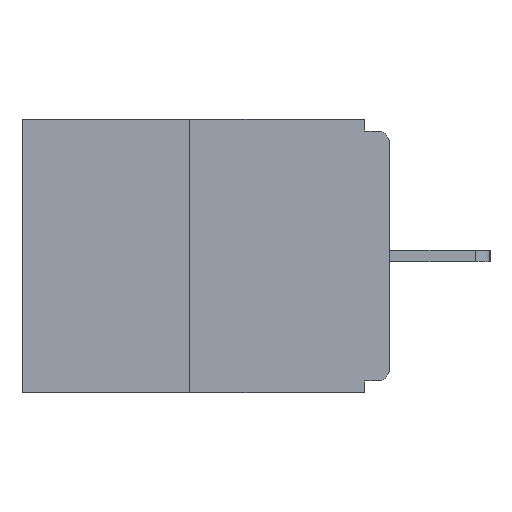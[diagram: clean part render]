
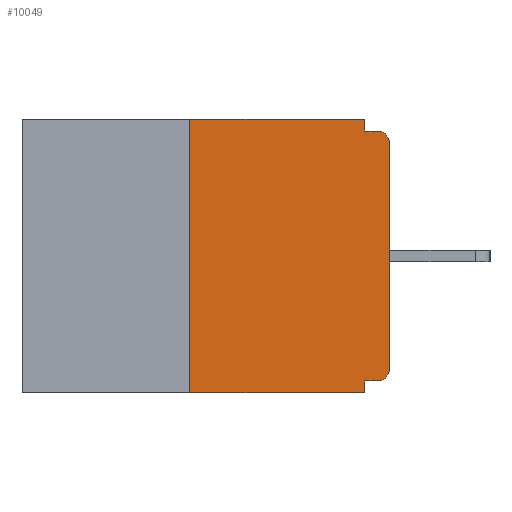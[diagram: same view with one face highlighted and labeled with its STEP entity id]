
A CAD part, left-side view. The second image highlights one B-rep face of the part: STEP entity #10049.
In plain terms, the highlighted planar face has unit normal (-1, 0, 0).
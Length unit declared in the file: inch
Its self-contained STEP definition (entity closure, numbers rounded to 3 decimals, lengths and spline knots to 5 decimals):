
#262 = LINE ( 'NONE', #20866, #19923 ) ;
#409 = EDGE_CURVE ( 'NONE', #17073, #11513, #262, .T. ) ;
#570 = CARTESIAN_POINT ( 'NONE',  ( 0., 0.015, -0.015 ) ) ;
#1238 = CARTESIAN_POINT ( 'NONE',  ( 0., 0.25, 0. ) ) ;
#2079 = LINE ( 'NONE', #9654, #21127 ) ;
#2628 = ORIENTED_EDGE ( 'NONE', *, *, #21669, .F. ) ;
#2881 = CARTESIAN_POINT ( 'NONE',  ( 0., 0.031, -0.343 ) ) ;
#2946 = AXIS2_PLACEMENT_3D ( 'NONE', #9299, #22091, #11186 ) ;
#3404 = DIRECTION ( 'NONE',  ( 0., 0., -1. ) ) ;
#3660 = LINE ( 'NONE', #16465, #13060 ) ;
#4600 = DIRECTION ( 'NONE',  ( 0., -1., 0. ) ) ;
#4614 = EDGE_CURVE ( 'NONE', #7440, #17073, #14393, .T. ) ;
#5332 = DIRECTION ( 'NONE',  ( 0., -1., 0. ) ) ;
#5369 = DIRECTION ( 'NONE',  ( 0., -1., 0. ) ) ;
#6088 = CARTESIAN_POINT ( 'NONE',  ( 0., 0., -0.313 ) ) ;
#6449 = CARTESIAN_POINT ( 'NONE',  ( 0., 0.031, -0.015 ) ) ;
#6926 = CARTESIAN_POINT ( 'NONE',  ( 0., 0.031, 0. ) ) ;
#7405 = EDGE_CURVE ( 'NONE', #10400, #9303, #20586, .T. ) ;
#7440 = VERTEX_POINT ( 'NONE', #12117 ) ;
#7557 = VERTEX_POINT ( 'NONE', #8673 ) ;
#7775 = LINE ( 'NONE', #13926, #21281 ) ;
#7869 = ORIENTED_EDGE ( 'NONE', *, *, #21294, .T. ) ;
#8654 = CARTESIAN_POINT ( 'NONE',  ( 0., 0.031, -0.328 ) ) ;
#8673 = CARTESIAN_POINT ( 'NONE',  ( 0., 0., -0.03 ) ) ;
#8986 = EDGE_CURVE ( 'NONE', #15023, #16984, #2079, .T. ) ;
#9113 = CARTESIAN_POINT ( 'NONE',  ( 0., 0.46, 0. ) ) ;
#9299 = CARTESIAN_POINT ( 'NONE',  ( 0., 0.015, -0.313 ) ) ;
#9303 = VERTEX_POINT ( 'NONE', #1238 ) ;
#9559 = DIRECTION ( 'NONE',  ( -1., 0., 0. ) ) ;
#9654 = CARTESIAN_POINT ( 'NONE',  ( 0., 0.031, 0. ) ) ;
#10049 = ADVANCED_FACE ( 'NONE', ( #13450 ), #19945, .F. ) ;
#10400 = VERTEX_POINT ( 'NONE', #11899 ) ;
#10853 = ORIENTED_EDGE ( 'NONE', *, *, #8986, .F. ) ;
#10904 = VECTOR ( 'NONE', #13775, 39.37008 ) ;
#11186 = DIRECTION ( 'NONE',  ( 0., 0., -1. ) ) ;
#11513 = VERTEX_POINT ( 'NONE', #2881 ) ;
#11641 = EDGE_LOOP ( 'NONE', ( #2628, #18586, #19138, #20249, #16054, #21385, #7869, #14059, #19420, #10853 ) ) ;
#11763 = CARTESIAN_POINT ( 'NONE',  ( 0., 0., 0. ) ) ;
#11899 = CARTESIAN_POINT ( 'NONE',  ( 0., 0.25, -0.343 ) ) ;
#12117 = CARTESIAN_POINT ( 'NONE',  ( 0., 0.015, -0.328 ) ) ;
#12666 = VECTOR ( 'NONE', #13659, 39.37008 ) ;
#12760 = CARTESIAN_POINT ( 'NONE',  ( 0., 0.46, 0. ) ) ;
#13060 = VECTOR ( 'NONE', #5332, 39.37008 ) ;
#13135 = VERTEX_POINT ( 'NONE', #6088 ) ;
#13450 = FACE_OUTER_BOUND ( 'NONE', #11641, .T. ) ;
#13659 = DIRECTION ( 'NONE',  ( 0., 0., 1. ) ) ;
#13669 = CARTESIAN_POINT ( 'NONE',  ( 0., 0.25, 0. ) ) ;
#13775 = DIRECTION ( 'NONE',  ( 0., 0., 1. ) ) ;
#13926 = CARTESIAN_POINT ( 'NONE',  ( 0., 0.46, -0.343 ) ) ;
#14059 = ORIENTED_EDGE ( 'NONE', *, *, #14738, .T. ) ;
#14393 = LINE ( 'NONE', #18410, #19193 ) ;
#14589 = DIRECTION ( 'NONE',  ( 1., 0., 0. ) ) ;
#14738 = EDGE_CURVE ( 'NONE', #7557, #21303, #22467, .T. ) ;
#14930 = LINE ( 'NONE', #9113, #18614 ) ;
#15023 = VERTEX_POINT ( 'NONE', #6926 ) ;
#15191 = EDGE_CURVE ( 'NONE', #7440, #13135, #17683, .T. ) ;
#16054 = ORIENTED_EDGE ( 'NONE', *, *, #4614, .F. ) ;
#16116 = EDGE_CURVE ( 'NONE', #10400, #11513, #7775, .T. ) ;
#16465 = CARTESIAN_POINT ( 'NONE',  ( 0., 0., -0.015 ) ) ;
#16724 = EDGE_CURVE ( 'NONE', #16984, #21303, #3660, .T. ) ;
#16984 = VERTEX_POINT ( 'NONE', #6449 ) ;
#17073 = VERTEX_POINT ( 'NONE', #8654 ) ;
#17098 = DIRECTION ( 'NONE',  ( 0., 0., -1. ) ) ;
#17578 = AXIS2_PLACEMENT_3D ( 'NONE', #20527, #9559, #22343 ) ;
#17683 = CIRCLE ( 'NONE', #2946, 0.015 ) ;
#18410 = CARTESIAN_POINT ( 'NONE',  ( 0., 0., -0.328 ) ) ;
#18586 = ORIENTED_EDGE ( 'NONE', *, *, #7405, .F. ) ;
#18614 = VECTOR ( 'NONE', #5369, 39.37008 ) ;
#19138 = ORIENTED_EDGE ( 'NONE', *, *, #16116, .T. ) ;
#19193 = VECTOR ( 'NONE', #20869, 39.37008 ) ;
#19420 = ORIENTED_EDGE ( 'NONE', *, *, #16724, .F. ) ;
#19923 = VECTOR ( 'NONE', #23584, 39.37008 ) ;
#19945 = PLANE ( 'NONE',  #20525 ) ;
#20249 = ORIENTED_EDGE ( 'NONE', *, *, #409, .F. ) ;
#20525 = AXIS2_PLACEMENT_3D ( 'NONE', #12760, #14589, #3404 ) ;
#20527 = CARTESIAN_POINT ( 'NONE',  ( 0., 0.015, -0.03 ) ) ;
#20586 = LINE ( 'NONE', #13669, #10904 ) ;
#20866 = CARTESIAN_POINT ( 'NONE',  ( 0., 0.031, -0.343 ) ) ;
#20869 = DIRECTION ( 'NONE',  ( 0., 1., 0. ) ) ;
#21127 = VECTOR ( 'NONE', #17098, 39.37008 ) ;
#21281 = VECTOR ( 'NONE', #4600, 39.37008 ) ;
#21294 = EDGE_CURVE ( 'NONE', #13135, #7557, #22839, .T. ) ;
#21303 = VERTEX_POINT ( 'NONE', #570 ) ;
#21385 = ORIENTED_EDGE ( 'NONE', *, *, #15191, .T. ) ;
#21669 = EDGE_CURVE ( 'NONE', #9303, #15023, #14930, .T. ) ;
#22091 = DIRECTION ( 'NONE',  ( -1., 0., 0. ) ) ;
#22343 = DIRECTION ( 'NONE',  ( 0., 0., -1. ) ) ;
#22467 = CIRCLE ( 'NONE', #17578, 0.015 ) ;
#22839 = LINE ( 'NONE', #11763, #12666 ) ;
#23584 = DIRECTION ( 'NONE',  ( 0., 0., -1. ) ) ;
